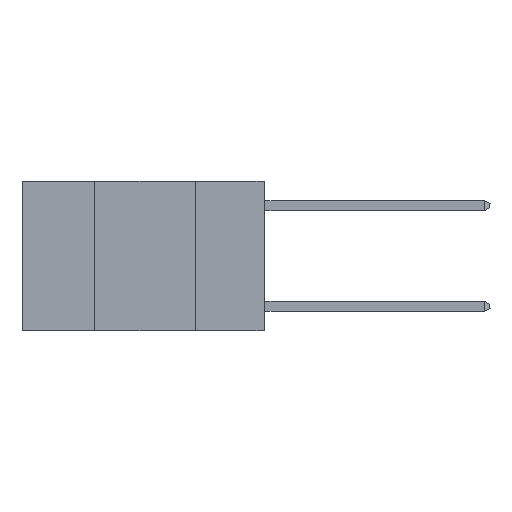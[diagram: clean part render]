
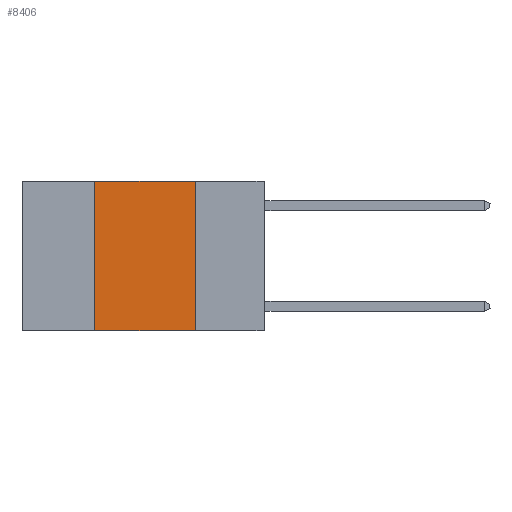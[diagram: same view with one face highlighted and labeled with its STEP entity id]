
A CAD part, left-side view. The second image highlights one B-rep face of the part: STEP entity #8406.
In plain terms, the highlighted planar face has unit normal (-1, 0, 0).
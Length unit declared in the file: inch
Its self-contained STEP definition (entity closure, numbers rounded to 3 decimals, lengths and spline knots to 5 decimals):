
#92 = CARTESIAN_POINT ( 'NONE',  ( 0., 0.6, -0.37 ) ) ;
#230 = CARTESIAN_POINT ( 'NONE',  ( 0., 0.42, -0.37 ) ) ;
#778 = DIRECTION ( 'NONE',  ( 0., 0., 1. ) ) ;
#830 = PLANE ( 'NONE',  #11554 ) ;
#1200 = EDGE_LOOP ( 'NONE', ( #2901, #19432, #5253, #6066 ) ) ;
#1456 = LINE ( 'NONE', #3162, #7776 ) ;
#1744 = LINE ( 'NONE', #92, #11651 ) ;
#2901 = ORIENTED_EDGE ( 'NONE', *, *, #13954, .F. ) ;
#3162 = CARTESIAN_POINT ( 'NONE',  ( 0., 0.17, 0. ) ) ;
#3463 = CARTESIAN_POINT ( 'NONE',  ( 0., 0.17, -0.37 ) ) ;
#4043 = CARTESIAN_POINT ( 'NONE',  ( 0., 0.6, 0. ) ) ;
#4539 = DIRECTION ( 'NONE',  ( 0., -1., 0. ) ) ;
#4541 = VERTEX_POINT ( 'NONE', #230 ) ;
#5253 = ORIENTED_EDGE ( 'NONE', *, *, #17713, .F. ) ;
#5652 = FACE_OUTER_BOUND ( 'NONE', #1200, .T. ) ;
#5955 = EDGE_CURVE ( 'NONE', #4541, #7115, #1744, .T. ) ;
#6066 = ORIENTED_EDGE ( 'NONE', *, *, #5955, .T. ) ;
#6735 = CARTESIAN_POINT ( 'NONE',  ( 0., 0.17, 0. ) ) ;
#7115 = VERTEX_POINT ( 'NONE', #3463 ) ;
#7359 = DIRECTION ( 'NONE',  ( 1., 0., 0. ) ) ;
#7776 = VECTOR ( 'NONE', #21124, 39.37008 ) ;
#8406 = ADVANCED_FACE ( 'NONE', ( #5652 ), #830, .F. ) ;
#9135 = CARTESIAN_POINT ( 'NONE',  ( 0., 0.42, 0. ) ) ;
#10612 = VECTOR ( 'NONE', #778, 39.37008 ) ;
#10905 = LINE ( 'NONE', #15976, #16366 ) ;
#11554 = AXIS2_PLACEMENT_3D ( 'NONE', #4043, #7359, #15126 ) ;
#11651 = VECTOR ( 'NONE', #14842, 39.37008 ) ;
#12263 = LINE ( 'NONE', #9135, #10612 ) ;
#13094 = CARTESIAN_POINT ( 'NONE',  ( 0., 0.42, 0. ) ) ;
#13708 = EDGE_CURVE ( 'NONE', #19740, #21241, #10905, .T. ) ;
#13954 = EDGE_CURVE ( 'NONE', #21241, #7115, #1456, .T. ) ;
#14842 = DIRECTION ( 'NONE',  ( 0., -1., 0. ) ) ;
#15126 = DIRECTION ( 'NONE',  ( 0., 0., -1. ) ) ;
#15976 = CARTESIAN_POINT ( 'NONE',  ( 0., 0.6, 0. ) ) ;
#16366 = VECTOR ( 'NONE', #4539, 39.37008 ) ;
#17713 = EDGE_CURVE ( 'NONE', #4541, #19740, #12263, .T. ) ;
#19432 = ORIENTED_EDGE ( 'NONE', *, *, #13708, .F. ) ;
#19740 = VERTEX_POINT ( 'NONE', #13094 ) ;
#21124 = DIRECTION ( 'NONE',  ( 0., 0., -1. ) ) ;
#21241 = VERTEX_POINT ( 'NONE', #6735 ) ;
